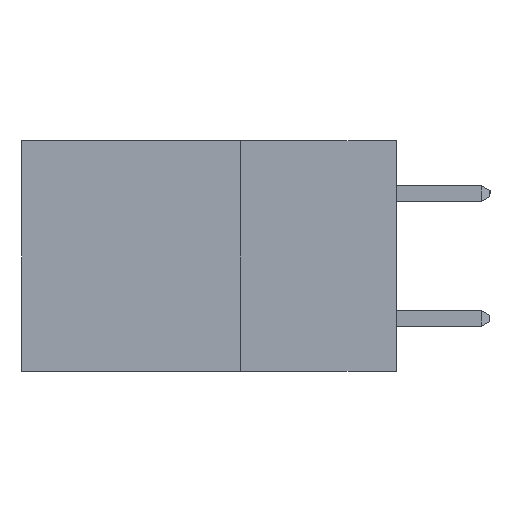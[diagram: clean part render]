
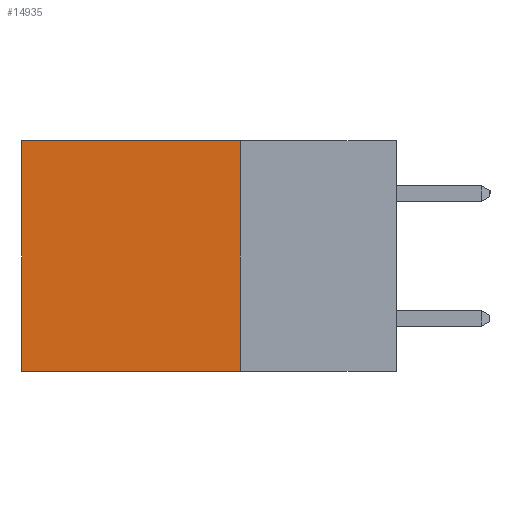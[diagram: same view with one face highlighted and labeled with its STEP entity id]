
A CAD part, left-side view. The second image highlights one B-rep face of the part: STEP entity #14935.
In plain terms, the highlighted planar face has unit normal (-1, 0, 0).
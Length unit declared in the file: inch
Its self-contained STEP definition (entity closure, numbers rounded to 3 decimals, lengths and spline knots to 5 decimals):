
#1614 = EDGE_CURVE ( 'NONE', #25022, #5338, #19913, .T. ) ;
#3289 = LINE ( 'NONE', #22439, #8226 ) ;
#3918 = CARTESIAN_POINT ( 'NONE',  ( 0.2615, 0.25, -0.37 ) ) ;
#5338 = VERTEX_POINT ( 'NONE', #10043 ) ;
#5809 = VERTEX_POINT ( 'NONE', #3918 ) ;
#6022 = ORIENTED_EDGE ( 'NONE', *, *, #23847, .T. ) ;
#6348 = FACE_OUTER_BOUND ( 'NONE', #21300, .T. ) ;
#6610 = DIRECTION ( 'NONE',  ( 0., 0., -1. ) ) ;
#7846 = LINE ( 'NONE', #17858, #11969 ) ;
#8226 = VECTOR ( 'NONE', #21110, 39.37008 ) ;
#9208 = CARTESIAN_POINT ( 'NONE',  ( 0.2615, 0.6, -0.37 ) ) ;
#10043 = CARTESIAN_POINT ( 'NONE',  ( 0.2615, 0.6, 0. ) ) ;
#11969 = VECTOR ( 'NONE', #11991, 39.37008 ) ;
#11991 = DIRECTION ( 'NONE',  ( 0., 0., -1. ) ) ;
#12341 = PLANE ( 'NONE',  #12679 ) ;
#12356 = DIRECTION ( 'NONE',  ( 0., 1., 0. ) ) ;
#12679 = AXIS2_PLACEMENT_3D ( 'NONE', #16507, #24446, #6610 ) ;
#12682 = ORIENTED_EDGE ( 'NONE', *, *, #25378, .F. ) ;
#13083 = CARTESIAN_POINT ( 'NONE',  ( 0.2615, 0.25, 0. ) ) ;
#13845 = CARTESIAN_POINT ( 'NONE',  ( 0.2615, 0.25, -0.37 ) ) ;
#14935 = ADVANCED_FACE ( 'NONE', ( #6348 ), #12341, .F. ) ;
#16507 = CARTESIAN_POINT ( 'NONE',  ( 0.2615, 0.25, -0.37 ) ) ;
#17345 = VECTOR ( 'NONE', #19842, 39.37008 ) ;
#17753 = VERTEX_POINT ( 'NONE', #9208 ) ;
#17858 = CARTESIAN_POINT ( 'NONE',  ( 0.2615, 0.6, -0.37 ) ) ;
#18047 = ORIENTED_EDGE ( 'NONE', *, *, #21664, .F. ) ;
#19150 = VECTOR ( 'NONE', #12356, 39.37008 ) ;
#19842 = DIRECTION ( 'NONE',  ( 0., 1., 0. ) ) ;
#19913 = LINE ( 'NONE', #22122, #19150 ) ;
#21110 = DIRECTION ( 'NONE',  ( 0., 0., -1. ) ) ;
#21300 = EDGE_LOOP ( 'NONE', ( #6022, #18047, #12682, #22816 ) ) ;
#21664 = EDGE_CURVE ( 'NONE', #5809, #17753, #21929, .T. ) ;
#21929 = LINE ( 'NONE', #13845, #17345 ) ;
#22122 = CARTESIAN_POINT ( 'NONE',  ( 0.2615, 0.25, 0. ) ) ;
#22439 = CARTESIAN_POINT ( 'NONE',  ( 0.2615, 0.25, -0.37 ) ) ;
#22816 = ORIENTED_EDGE ( 'NONE', *, *, #1614, .T. ) ;
#23847 = EDGE_CURVE ( 'NONE', #5338, #17753, #7846, .T. ) ;
#24446 = DIRECTION ( 'NONE',  ( 1., 0., 0. ) ) ;
#25022 = VERTEX_POINT ( 'NONE', #13083 ) ;
#25378 = EDGE_CURVE ( 'NONE', #25022, #5809, #3289, .T. ) ;
